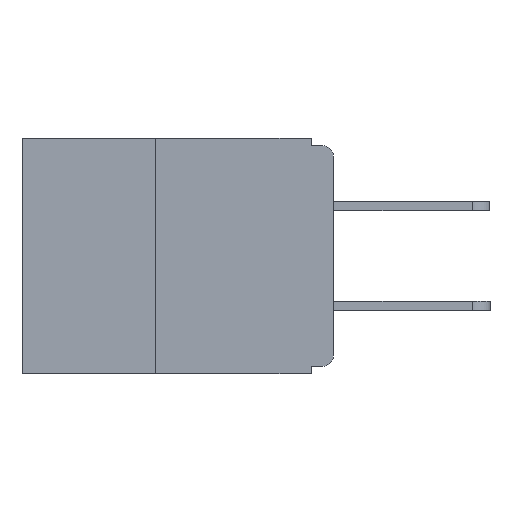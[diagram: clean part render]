
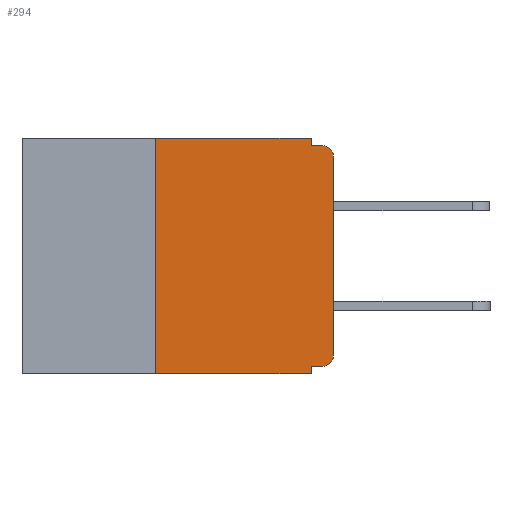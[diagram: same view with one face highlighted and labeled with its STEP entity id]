
A CAD part, left-side view. The second image highlights one B-rep face of the part: STEP entity #294.
In plain terms, the highlighted planar face has unit normal (-1, 0, 0).
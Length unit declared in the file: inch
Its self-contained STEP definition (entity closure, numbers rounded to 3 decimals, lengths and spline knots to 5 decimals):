
#294 = ADVANCED_FACE ( 'NONE', ( #16839 ), #2768, .F. ) ;
#923 = CARTESIAN_POINT ( 'NONE',  ( 0., 0.25, 0. ) ) ;
#1042 = DIRECTION ( 'NONE',  ( 0., 0., 1. ) ) ;
#2176 = DIRECTION ( 'NONE',  ( 0., 0., -1. ) ) ;
#2394 = CARTESIAN_POINT ( 'NONE',  ( 0., 0.25, -0.33 ) ) ;
#2768 = PLANE ( 'NONE',  #18576 ) ;
#2804 = DIRECTION ( 'NONE',  ( 0., -1., 0. ) ) ;
#3019 = CARTESIAN_POINT ( 'NONE',  ( 0., 0., -0.01 ) ) ;
#3077 = CIRCLE ( 'NONE', #23843, 0.015 ) ;
#3084 = EDGE_CURVE ( 'NONE', #30402, #24833, #10088, .T. ) ;
#3829 = DIRECTION ( 'NONE',  ( 0., 0., -1. ) ) ;
#4625 = CARTESIAN_POINT ( 'NONE',  ( 0., 0.031, 0. ) ) ;
#5609 = VECTOR ( 'NONE', #27457, 39.37008 ) ;
#6145 = CARTESIAN_POINT ( 'NONE',  ( 0., 0.031, -0.33 ) ) ;
#6522 = DIRECTION ( 'NONE',  ( 0., 1., 0. ) ) ;
#6628 = VERTEX_POINT ( 'NONE', #32491 ) ;
#6766 = ORIENTED_EDGE ( 'NONE', *, *, #10859, .F. ) ;
#6929 = VECTOR ( 'NONE', #27177, 39.37008 ) ;
#7839 = CARTESIAN_POINT ( 'NONE',  ( 0., 0.015, -0.32 ) ) ;
#8047 = VERTEX_POINT ( 'NONE', #32138 ) ;
#8113 = VECTOR ( 'NONE', #6522, 39.37008 ) ;
#8187 = ORIENTED_EDGE ( 'NONE', *, *, #23723, .T. ) ;
#8532 = LINE ( 'NONE', #22205, #15591 ) ;
#8993 = DIRECTION ( 'NONE',  ( -1., 0., 0. ) ) ;
#9289 = ORIENTED_EDGE ( 'NONE', *, *, #31097, .F. ) ;
#9502 = LINE ( 'NONE', #24098, #29990 ) ;
#10088 = LINE ( 'NONE', #33074, #30532 ) ;
#10515 = CARTESIAN_POINT ( 'NONE',  ( 0., 0., 0. ) ) ;
#10859 = EDGE_CURVE ( 'NONE', #22678, #30402, #9502, .T. ) ;
#11806 = CARTESIAN_POINT ( 'NONE',  ( 0., 0.031, 0. ) ) ;
#12681 = VERTEX_POINT ( 'NONE', #7839 ) ;
#12910 = ORIENTED_EDGE ( 'NONE', *, *, #19100, .T. ) ;
#13029 = EDGE_LOOP ( 'NONE', ( #12910, #33225, #23189, #17643, #27861, #6766, #8187, #9289, #16194, #15569 ) ) ;
#15100 = DIRECTION ( 'NONE',  ( -1., 0., 0. ) ) ;
#15569 = ORIENTED_EDGE ( 'NONE', *, *, #15712, .T. ) ;
#15591 = VECTOR ( 'NONE', #3829, 39.37008 ) ;
#15712 = EDGE_CURVE ( 'NONE', #12681, #16017, #3077, .T. ) ;
#15865 = VECTOR ( 'NONE', #26488, 39.37008 ) ;
#16017 = VERTEX_POINT ( 'NONE', #26491 ) ;
#16194 = ORIENTED_EDGE ( 'NONE', *, *, #23647, .F. ) ;
#16839 = FACE_OUTER_BOUND ( 'NONE', #13029, .T. ) ;
#17392 = EDGE_CURVE ( 'NONE', #32207, #8047, #18720, .T. ) ;
#17643 = ORIENTED_EDGE ( 'NONE', *, *, #23000, .F. ) ;
#18576 = AXIS2_PLACEMENT_3D ( 'NONE', #20039, #31052, #2176 ) ;
#18720 = CIRCLE ( 'NONE', #29093, 0.015 ) ;
#19100 = EDGE_CURVE ( 'NONE', #16017, #32207, #20743, .T. ) ;
#19665 = LINE ( 'NONE', #22438, #5609 ) ;
#20039 = CARTESIAN_POINT ( 'NONE',  ( 0., 0.437, 0. ) ) ;
#20743 = LINE ( 'NONE', #10515, #33287 ) ;
#21270 = LINE ( 'NONE', #24756, #8113 ) ;
#21723 = LINE ( 'NONE', #11806, #6929 ) ;
#22205 = CARTESIAN_POINT ( 'NONE',  ( 0., 0.031, -0.33 ) ) ;
#22438 = CARTESIAN_POINT ( 'NONE',  ( 0., 0.437, -0.33 ) ) ;
#22678 = VERTEX_POINT ( 'NONE', #2394 ) ;
#22715 = LINE ( 'NONE', #3019, #15865 ) ;
#23000 = EDGE_CURVE ( 'NONE', #24833, #31103, #21723, .T. ) ;
#23189 = ORIENTED_EDGE ( 'NONE', *, *, #26201, .F. ) ;
#23647 = EDGE_CURVE ( 'NONE', #12681, #6628, #21270, .T. ) ;
#23723 = EDGE_CURVE ( 'NONE', #22678, #24554, #19665, .T. ) ;
#23843 = AXIS2_PLACEMENT_3D ( 'NONE', #30320, #15100, #32845 ) ;
#24098 = CARTESIAN_POINT ( 'NONE',  ( 0., 0.25, -0.33 ) ) ;
#24554 = VERTEX_POINT ( 'NONE', #6145 ) ;
#24558 = CARTESIAN_POINT ( 'NONE',  ( 0., 0.015, -0.025 ) ) ;
#24756 = CARTESIAN_POINT ( 'NONE',  ( 0., 0., -0.32 ) ) ;
#24833 = VERTEX_POINT ( 'NONE', #4625 ) ;
#25977 = DIRECTION ( 'NONE',  ( 0., 0., 1. ) ) ;
#26201 = EDGE_CURVE ( 'NONE', #31103, #8047, #22715, .T. ) ;
#26488 = DIRECTION ( 'NONE',  ( 0., -1., 0. ) ) ;
#26491 = CARTESIAN_POINT ( 'NONE',  ( 0., 0., -0.305 ) ) ;
#27065 = DIRECTION ( 'NONE',  ( 0., 0., -1. ) ) ;
#27177 = DIRECTION ( 'NONE',  ( 0., 0., -1. ) ) ;
#27218 = CARTESIAN_POINT ( 'NONE',  ( 0., 0.031, -0.01 ) ) ;
#27457 = DIRECTION ( 'NONE',  ( 0., -1., 0. ) ) ;
#27861 = ORIENTED_EDGE ( 'NONE', *, *, #3084, .F. ) ;
#28903 = CARTESIAN_POINT ( 'NONE',  ( 0., 0., -0.025 ) ) ;
#29093 = AXIS2_PLACEMENT_3D ( 'NONE', #24558, #8993, #27065 ) ;
#29990 = VECTOR ( 'NONE', #1042, 39.37008 ) ;
#30320 = CARTESIAN_POINT ( 'NONE',  ( 0., 0.015, -0.305 ) ) ;
#30402 = VERTEX_POINT ( 'NONE', #923 ) ;
#30532 = VECTOR ( 'NONE', #2804, 39.37008 ) ;
#31052 = DIRECTION ( 'NONE',  ( 1., 0., 0. ) ) ;
#31097 = EDGE_CURVE ( 'NONE', #6628, #24554, #8532, .T. ) ;
#31103 = VERTEX_POINT ( 'NONE', #27218 ) ;
#32138 = CARTESIAN_POINT ( 'NONE',  ( 0., 0.015, -0.01 ) ) ;
#32207 = VERTEX_POINT ( 'NONE', #28903 ) ;
#32491 = CARTESIAN_POINT ( 'NONE',  ( 0., 0.031, -0.32 ) ) ;
#32845 = DIRECTION ( 'NONE',  ( 0., 0., -1. ) ) ;
#33074 = CARTESIAN_POINT ( 'NONE',  ( 0., 0.437, 0. ) ) ;
#33225 = ORIENTED_EDGE ( 'NONE', *, *, #17392, .T. ) ;
#33287 = VECTOR ( 'NONE', #25977, 39.37008 ) ;
